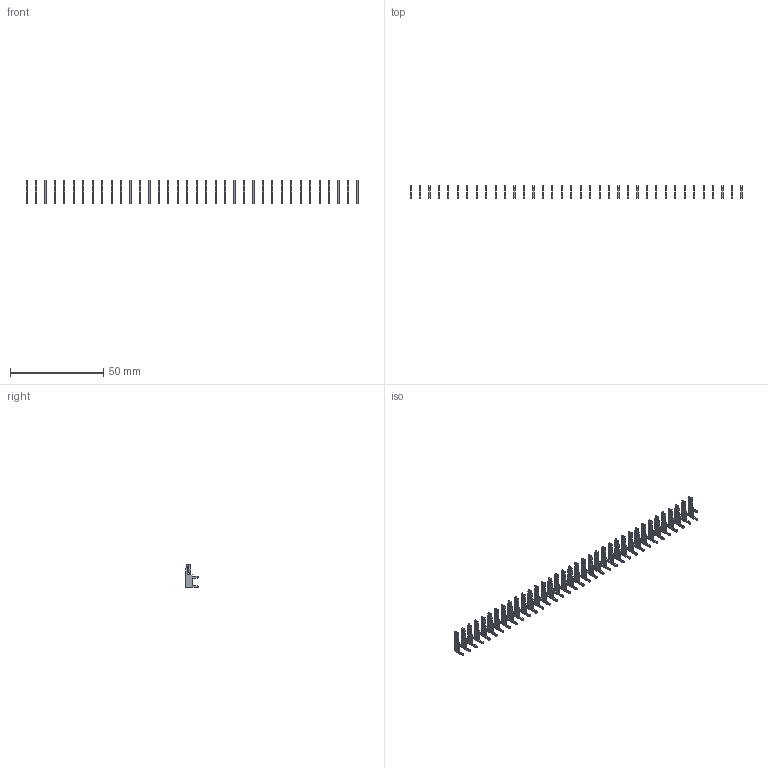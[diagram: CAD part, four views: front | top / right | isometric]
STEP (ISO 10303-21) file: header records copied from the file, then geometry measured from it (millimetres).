
FILE_DESCRIPTION (( 'STEP AP203' ), '1' );
FILE_NAME ('105-036-203-200.STEP', '2020-08-29T23:43:40', ( '' ), ( '' ), 'SwSTEP 2.0', 'SolidWorks 2020', '' );
FILE_SCHEMA (( 'CONFIG_CONTROL_DESIGN' ));
Length unit declared in the file: inch
Products named in the file (2): 105-036-203-200; 100-290-001_100-290-203
Assembly tree (36 placements, depth 2):
  105-036-203-200
    100-290-001_100-290-203  x36
Bounding box: 178.4 x 6.53 x 12.7 mm (x, y, z)
Volume: 908.8 mm3; surface area: 4165.9 mm2
Topology: 36 solids, 36 shells, 1008 faces, 2808 edges, 1872 vertices
Faces by surface type: plane 756, cylinder 252
Entity records: 2216 total; most frequent: DIRECTION 222, CARTESIAN_POINT 209, ORIENTED_EDGE 156, LOCAL_TIME 82, DATE_AND_TIME 82, COORDINATED_UNIVERSAL_TIME_OFFSET 82, CALENDAR_DATE 82, AXIS2_PLACEMENT_3D 81
